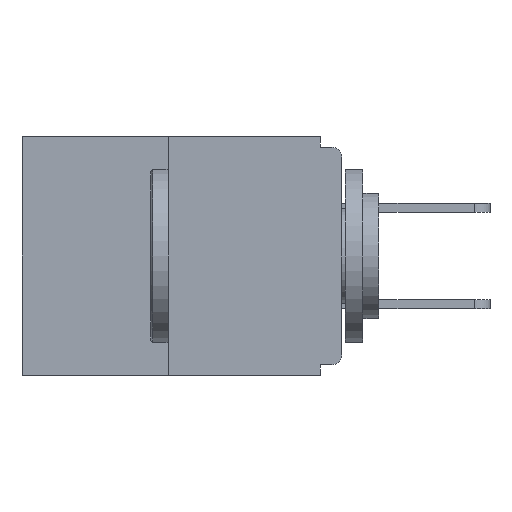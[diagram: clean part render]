
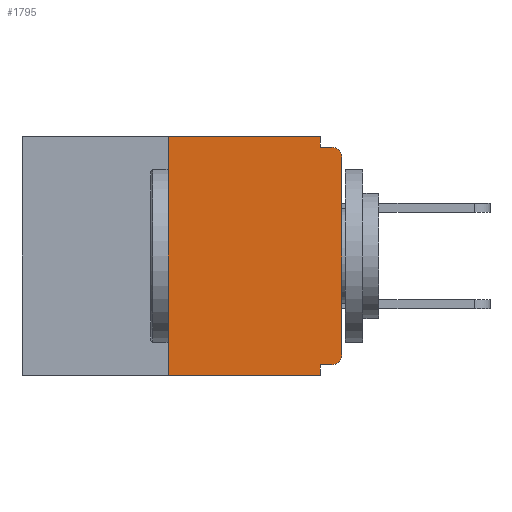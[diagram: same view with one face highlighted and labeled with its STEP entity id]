
A CAD part, left-side view. The second image highlights one B-rep face of the part: STEP entity #1795.
In plain terms, the highlighted planar face has unit normal (-1, 0, 0).
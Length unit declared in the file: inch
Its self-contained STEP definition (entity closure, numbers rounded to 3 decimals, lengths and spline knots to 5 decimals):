
#41 = EDGE_CURVE ( 'NONE', #5415, #3754, #1119, .T. ) ;
#301 = LINE ( 'NONE', #5954, #2016 ) ;
#309 = ORIENTED_EDGE ( 'NONE', *, *, #1381, .F. ) ;
#319 = CARTESIAN_POINT ( 'NONE',  ( 0., 0.015, -0.328 ) ) ;
#538 = CIRCLE ( 'NONE', #9964, 0.015 ) ;
#561 = FACE_OUTER_BOUND ( 'NONE', #10263, .T. ) ;
#661 = EDGE_CURVE ( 'NONE', #6386, #7505, #2548, .T. ) ;
#826 = LINE ( 'NONE', #1138, #3279 ) ;
#934 = DIRECTION ( 'NONE',  ( 0., 0., -1. ) ) ;
#979 = CARTESIAN_POINT ( 'NONE',  ( 0., 0.46, 0. ) ) ;
#1070 = DIRECTION ( 'NONE',  ( 0., 1., 0. ) ) ;
#1119 = LINE ( 'NONE', #2747, #9014 ) ;
#1138 = CARTESIAN_POINT ( 'NONE',  ( 0., 0.46, 0. ) ) ;
#1337 = EDGE_CURVE ( 'NONE', #11573, #10468, #8124, .T. ) ;
#1379 = CARTESIAN_POINT ( 'NONE',  ( 0., 0.031, -0.015 ) ) ;
#1381 = EDGE_CURVE ( 'NONE', #7404, #5854, #826, .T. ) ;
#1400 = EDGE_CURVE ( 'NONE', #6386, #11573, #538, .T. ) ;
#1571 = PLANE ( 'NONE',  #4901 ) ;
#1711 = DIRECTION ( 'NONE',  ( 0., -1., 0. ) ) ;
#1795 = ADVANCED_FACE ( 'NONE', ( #561 ), #1571, .F. ) ;
#1940 = DIRECTION ( 'NONE',  ( 0., -1., 0. ) ) ;
#1961 = VECTOR ( 'NONE', #10196, 39.37008 ) ;
#2016 = VECTOR ( 'NONE', #11443, 39.37008 ) ;
#2198 = EDGE_CURVE ( 'NONE', #5854, #6712, #301, .T. ) ;
#2548 = LINE ( 'NONE', #9219, #3420 ) ;
#2633 = CARTESIAN_POINT ( 'NONE',  ( 0., 0., -0.015 ) ) ;
#2747 = CARTESIAN_POINT ( 'NONE',  ( 0., 0.46, -0.343 ) ) ;
#2758 = CARTESIAN_POINT ( 'NONE',  ( 0., 0.031, 0. ) ) ;
#3057 = CARTESIAN_POINT ( 'NONE',  ( 0., 0.031, -0.343 ) ) ;
#3064 = CARTESIAN_POINT ( 'NONE',  ( 0., 0.25, -0.343 ) ) ;
#3233 = CARTESIAN_POINT ( 'NONE',  ( 0., 0.031, -0.328 ) ) ;
#3279 = VECTOR ( 'NONE', #1940, 39.37008 ) ;
#3420 = VECTOR ( 'NONE', #1070, 39.37008 ) ;
#3544 = ORIENTED_EDGE ( 'NONE', *, *, #8183, .T. ) ;
#3658 = ORIENTED_EDGE ( 'NONE', *, *, #661, .F. ) ;
#3754 = VERTEX_POINT ( 'NONE', #3057 ) ;
#3833 = CARTESIAN_POINT ( 'NONE',  ( 0., 0.015, -0.313 ) ) ;
#4383 = DIRECTION ( 'NONE',  ( 0., 0., -1. ) ) ;
#4470 = VECTOR ( 'NONE', #1711, 39.37008 ) ;
#4846 = DIRECTION ( 'NONE',  ( 0., 0., 1. ) ) ;
#4901 = AXIS2_PLACEMENT_3D ( 'NONE', #979, #8301, #4383 ) ;
#5006 = ORIENTED_EDGE ( 'NONE', *, *, #1337, .T. ) ;
#5106 = VERTEX_POINT ( 'NONE', #7341 ) ;
#5171 = AXIS2_PLACEMENT_3D ( 'NONE', #5516, #8297, #934 ) ;
#5243 = LINE ( 'NONE', #9211, #6644 ) ;
#5415 = VERTEX_POINT ( 'NONE', #3064 ) ;
#5516 = CARTESIAN_POINT ( 'NONE',  ( 0., 0.015, -0.03 ) ) ;
#5641 = CARTESIAN_POINT ( 'NONE',  ( 0., 0., 0. ) ) ;
#5814 = EDGE_CURVE ( 'NONE', #7505, #3754, #5243, .T. ) ;
#5854 = VERTEX_POINT ( 'NONE', #2758 ) ;
#5906 = EDGE_CURVE ( 'NONE', #5415, #7404, #8381, .T. ) ;
#5949 = CARTESIAN_POINT ( 'NONE',  ( 0., 0.25, 0. ) ) ;
#5954 = CARTESIAN_POINT ( 'NONE',  ( 0., 0.031, 0. ) ) ;
#6380 = DIRECTION ( 'NONE',  ( 0., 0., -1. ) ) ;
#6386 = VERTEX_POINT ( 'NONE', #319 ) ;
#6644 = VECTOR ( 'NONE', #6380, 39.37008 ) ;
#6712 = VERTEX_POINT ( 'NONE', #1379 ) ;
#6903 = VECTOR ( 'NONE', #4846, 39.37008 ) ;
#7156 = ORIENTED_EDGE ( 'NONE', *, *, #8804, .F. ) ;
#7341 = CARTESIAN_POINT ( 'NONE',  ( 0., 0.015, -0.015 ) ) ;
#7404 = VERTEX_POINT ( 'NONE', #5949 ) ;
#7505 = VERTEX_POINT ( 'NONE', #3233 ) ;
#7738 = LINE ( 'NONE', #2633, #4470 ) ;
#8124 = LINE ( 'NONE', #5641, #1961 ) ;
#8183 = EDGE_CURVE ( 'NONE', #10468, #5106, #11330, .T. ) ;
#8297 = DIRECTION ( 'NONE',  ( -1., 0., 0. ) ) ;
#8301 = DIRECTION ( 'NONE',  ( 1., 0., 0. ) ) ;
#8381 = LINE ( 'NONE', #10199, #6903 ) ;
#8484 = ORIENTED_EDGE ( 'NONE', *, *, #2198, .F. ) ;
#8804 = EDGE_CURVE ( 'NONE', #6712, #5106, #7738, .T. ) ;
#9014 = VECTOR ( 'NONE', #9274, 39.37008 ) ;
#9211 = CARTESIAN_POINT ( 'NONE',  ( 0., 0.031, -0.343 ) ) ;
#9219 = CARTESIAN_POINT ( 'NONE',  ( 0., 0., -0.328 ) ) ;
#9241 = DIRECTION ( 'NONE',  ( -1., 0., 0. ) ) ;
#9274 = DIRECTION ( 'NONE',  ( 0., -1., 0. ) ) ;
#9621 = ORIENTED_EDGE ( 'NONE', *, *, #5906, .F. ) ;
#9744 = CARTESIAN_POINT ( 'NONE',  ( 0., 0., -0.03 ) ) ;
#9826 = ORIENTED_EDGE ( 'NONE', *, *, #1400, .T. ) ;
#9964 = AXIS2_PLACEMENT_3D ( 'NONE', #3833, #9241, #11086 ) ;
#10196 = DIRECTION ( 'NONE',  ( 0., 0., 1. ) ) ;
#10199 = CARTESIAN_POINT ( 'NONE',  ( 0., 0.25, 0. ) ) ;
#10263 = EDGE_LOOP ( 'NONE', ( #309, #9621, #10901, #10361, #3658, #9826, #5006, #3544, #7156, #8484 ) ) ;
#10361 = ORIENTED_EDGE ( 'NONE', *, *, #5814, .F. ) ;
#10468 = VERTEX_POINT ( 'NONE', #9744 ) ;
#10863 = CARTESIAN_POINT ( 'NONE',  ( 0., 0., -0.313 ) ) ;
#10901 = ORIENTED_EDGE ( 'NONE', *, *, #41, .T. ) ;
#11086 = DIRECTION ( 'NONE',  ( 0., 0., -1. ) ) ;
#11330 = CIRCLE ( 'NONE', #5171, 0.015 ) ;
#11443 = DIRECTION ( 'NONE',  ( 0., 0., -1. ) ) ;
#11573 = VERTEX_POINT ( 'NONE', #10863 ) ;
